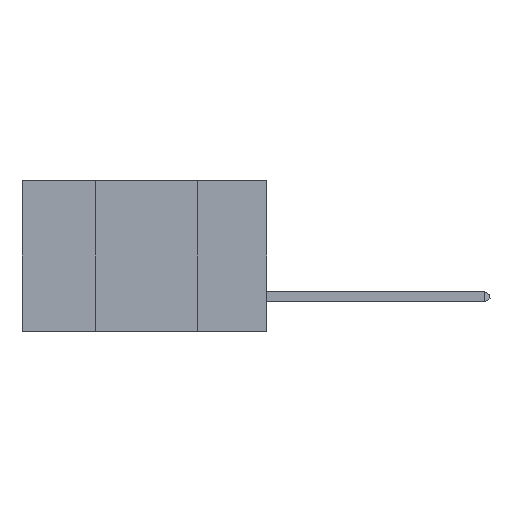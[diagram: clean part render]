
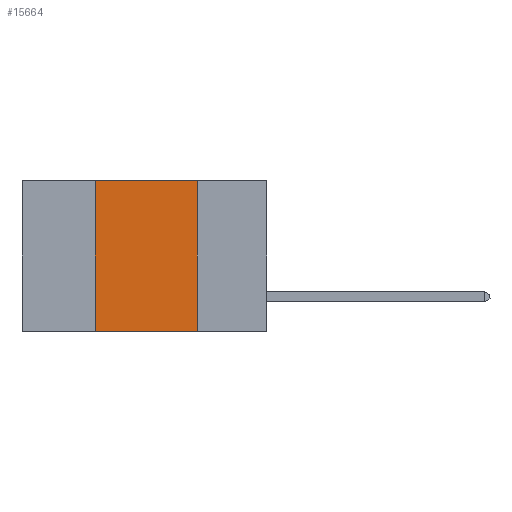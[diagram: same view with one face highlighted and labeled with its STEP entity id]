
A CAD part, left-side view. The second image highlights one B-rep face of the part: STEP entity #15664.
In plain terms, the highlighted planar face has unit normal (-1, 0, 0).
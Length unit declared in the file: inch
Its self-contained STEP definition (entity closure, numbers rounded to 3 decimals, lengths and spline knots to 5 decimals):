
#232 = CARTESIAN_POINT ( 'NONE',  ( 0., 0.17, 0. ) ) ;
#1683 = DIRECTION ( 'NONE',  ( 0., 0., -1. ) ) ;
#2546 = CARTESIAN_POINT ( 'NONE',  ( 0., 0.17, -0.37 ) ) ;
#3022 = LINE ( 'NONE', #31187, #25921 ) ;
#3092 = VECTOR ( 'NONE', #6431, 39.37008 ) ;
#3955 = EDGE_CURVE ( 'NONE', #32630, #28731, #28191, .T. ) ;
#4747 = CARTESIAN_POINT ( 'NONE',  ( 0., 0.6, 0. ) ) ;
#5447 = ORIENTED_EDGE ( 'NONE', *, *, #3955, .F. ) ;
#6295 = DIRECTION ( 'NONE',  ( 0., 0., -1. ) ) ;
#6431 = DIRECTION ( 'NONE',  ( 0., -1., 0. ) ) ;
#7594 = VECTOR ( 'NONE', #19686, 39.37008 ) ;
#7645 = VERTEX_POINT ( 'NONE', #25465 ) ;
#7772 = FACE_OUTER_BOUND ( 'NONE', #37190, .T. ) ;
#8684 = CARTESIAN_POINT ( 'NONE',  ( 0., 0.42, 0. ) ) ;
#11052 = LINE ( 'NONE', #24084, #3092 ) ;
#13359 = ORIENTED_EDGE ( 'NONE', *, *, #37872, .F. ) ;
#15255 = ORIENTED_EDGE ( 'NONE', *, *, #16305, .F. ) ;
#15354 = EDGE_CURVE ( 'NONE', #7645, #28731, #11052, .T. ) ;
#15664 = ADVANCED_FACE ( 'NONE', ( #7772 ), #34329, .F. ) ;
#16305 = EDGE_CURVE ( 'NONE', #7645, #29394, #3022, .T. ) ;
#19661 = DIRECTION ( 'NONE',  ( 1., 0., 0. ) ) ;
#19686 = DIRECTION ( 'NONE',  ( 0., -1., 0. ) ) ;
#20357 = VECTOR ( 'NONE', #6295, 39.37008 ) ;
#23627 = AXIS2_PLACEMENT_3D ( 'NONE', #37277, #19661, #1683 ) ;
#24084 = CARTESIAN_POINT ( 'NONE',  ( 0., 0.6, -0.37 ) ) ;
#25465 = CARTESIAN_POINT ( 'NONE',  ( 0., 0.42, -0.37 ) ) ;
#25921 = VECTOR ( 'NONE', #34121, 39.37008 ) ;
#28191 = LINE ( 'NONE', #232, #20357 ) ;
#28731 = VERTEX_POINT ( 'NONE', #2546 ) ;
#29050 = CARTESIAN_POINT ( 'NONE',  ( 0., 0.17, 0. ) ) ;
#29394 = VERTEX_POINT ( 'NONE', #8684 ) ;
#31048 = ORIENTED_EDGE ( 'NONE', *, *, #15354, .T. ) ;
#31187 = CARTESIAN_POINT ( 'NONE',  ( 0., 0.42, 0. ) ) ;
#31285 = LINE ( 'NONE', #4747, #7594 ) ;
#32630 = VERTEX_POINT ( 'NONE', #29050 ) ;
#34121 = DIRECTION ( 'NONE',  ( 0., 0., 1. ) ) ;
#34329 = PLANE ( 'NONE',  #23627 ) ;
#37190 = EDGE_LOOP ( 'NONE', ( #5447, #13359, #15255, #31048 ) ) ;
#37277 = CARTESIAN_POINT ( 'NONE',  ( 0., 0.6, 0. ) ) ;
#37872 = EDGE_CURVE ( 'NONE', #29394, #32630, #31285, .T. ) ;
